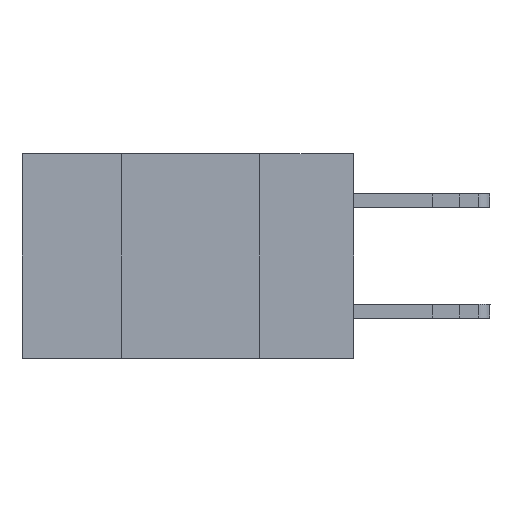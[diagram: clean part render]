
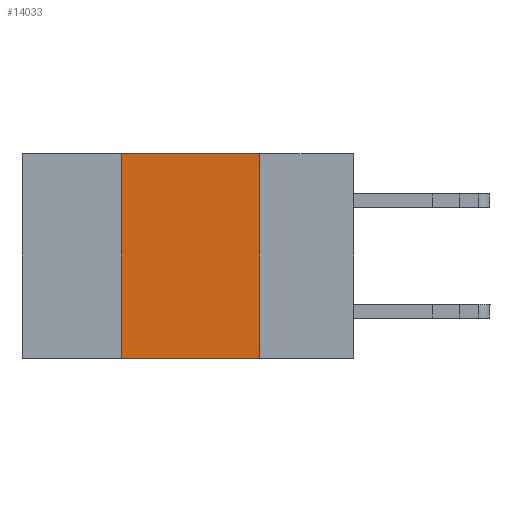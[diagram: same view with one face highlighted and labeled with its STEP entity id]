
A CAD part, left-side view. The second image highlights one B-rep face of the part: STEP entity #14033.
In plain terms, the highlighted planar face has unit normal (-1, 0, 0).
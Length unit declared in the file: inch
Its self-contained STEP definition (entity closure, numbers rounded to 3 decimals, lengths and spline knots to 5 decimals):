
#165 = VECTOR ( 'NONE', #16062, 39.37008 ) ;
#219 = AXIS2_PLACEMENT_3D ( 'NONE', #6935, #11391, #9164 ) ;
#568 = ORIENTED_EDGE ( 'NONE', *, *, #7468, .T. ) ;
#600 = ORIENTED_EDGE ( 'NONE', *, *, #9074, .F. ) ;
#995 = PLANE ( 'NONE',  #219 ) ;
#1127 = ORIENTED_EDGE ( 'NONE', *, *, #2751, .F. ) ;
#1633 = EDGE_CURVE ( 'NONE', #16235, #9801, #2597, .T. ) ;
#1975 = DIRECTION ( 'NONE',  ( 0., -1., 0. ) ) ;
#2597 = LINE ( 'NONE', #12571, #165 ) ;
#2751 = EDGE_CURVE ( 'NONE', #9801, #8306, #7710, .T. ) ;
#2803 = EDGE_LOOP ( 'NONE', ( #600, #1127, #7318, #568 ) ) ;
#3136 = LINE ( 'NONE', #3233, #13068 ) ;
#3233 = CARTESIAN_POINT ( 'NONE',  ( 0., 0.6, -0.37 ) ) ;
#3812 = LINE ( 'NONE', #14085, #14680 ) ;
#4217 = CARTESIAN_POINT ( 'NONE',  ( 0., 0.42, -0.37 ) ) ;
#5271 = DIRECTION ( 'NONE',  ( 0., 0., -1. ) ) ;
#6580 = CARTESIAN_POINT ( 'NONE',  ( 0., 0.42, 0. ) ) ;
#6935 = CARTESIAN_POINT ( 'NONE',  ( 0., 0.6, 0. ) ) ;
#7318 = ORIENTED_EDGE ( 'NONE', *, *, #1633, .F. ) ;
#7468 = EDGE_CURVE ( 'NONE', #16235, #11523, #3136, .T. ) ;
#7710 = LINE ( 'NONE', #15032, #12913 ) ;
#8306 = VERTEX_POINT ( 'NONE', #10483 ) ;
#9074 = EDGE_CURVE ( 'NONE', #8306, #11523, #3812, .T. ) ;
#9164 = DIRECTION ( 'NONE',  ( 0., 0., -1. ) ) ;
#9801 = VERTEX_POINT ( 'NONE', #6580 ) ;
#10483 = CARTESIAN_POINT ( 'NONE',  ( 0., 0.17, 0. ) ) ;
#10931 = CARTESIAN_POINT ( 'NONE',  ( 0., 0.17, -0.37 ) ) ;
#11391 = DIRECTION ( 'NONE',  ( 1., 0., 0. ) ) ;
#11523 = VERTEX_POINT ( 'NONE', #10931 ) ;
#12571 = CARTESIAN_POINT ( 'NONE',  ( 0., 0.42, 0. ) ) ;
#12913 = VECTOR ( 'NONE', #15324, 39.37008 ) ;
#13068 = VECTOR ( 'NONE', #1975, 39.37008 ) ;
#14033 = ADVANCED_FACE ( 'NONE', ( #14350 ), #995, .F. ) ;
#14085 = CARTESIAN_POINT ( 'NONE',  ( 0., 0.17, 0. ) ) ;
#14350 = FACE_OUTER_BOUND ( 'NONE', #2803, .T. ) ;
#14680 = VECTOR ( 'NONE', #5271, 39.37008 ) ;
#15032 = CARTESIAN_POINT ( 'NONE',  ( 0., 0.6, 0. ) ) ;
#15324 = DIRECTION ( 'NONE',  ( 0., -1., 0. ) ) ;
#16062 = DIRECTION ( 'NONE',  ( 0., 0., 1. ) ) ;
#16235 = VERTEX_POINT ( 'NONE', #4217 ) ;
